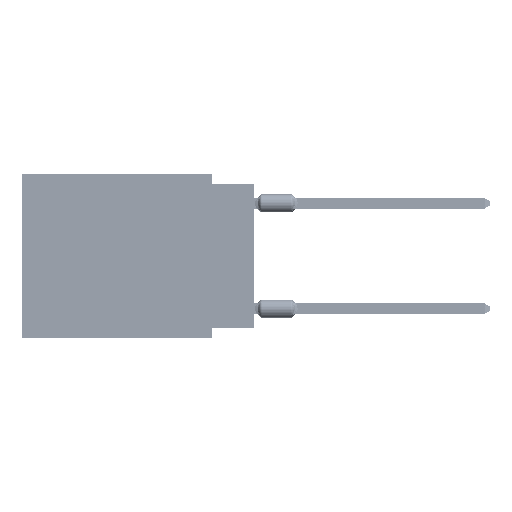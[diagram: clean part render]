
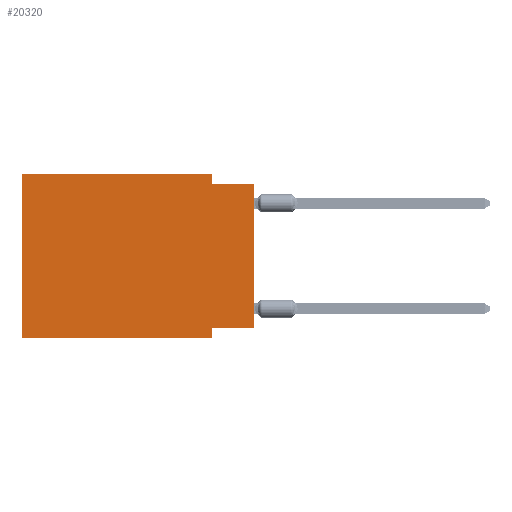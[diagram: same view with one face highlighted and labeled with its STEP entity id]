
A CAD part, left-side view. The second image highlights one B-rep face of the part: STEP entity #20320.
In plain terms, the highlighted planar face has unit normal (-1, 0, 0).
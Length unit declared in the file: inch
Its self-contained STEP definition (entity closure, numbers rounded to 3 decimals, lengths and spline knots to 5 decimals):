
#220 = DIRECTION ( 'NONE',  ( 0., -1., 0. ) ) ;
#3624 = EDGE_CURVE ( 'NONE', #69415, #12185, #21627, .T. ) ;
#5870 = EDGE_CURVE ( 'NONE', #60290, #19445, #73942, .T. ) ;
#5998 = LINE ( 'NONE', #48182, #35065 ) ;
#10390 = VECTOR ( 'NONE', #67314, 39.37008 ) ;
#12185 = VERTEX_POINT ( 'NONE', #50914 ) ;
#12834 = EDGE_CURVE ( 'NONE', #14353, #69415, #37160, .T. ) ;
#13113 = VECTOR ( 'NONE', #46015, 39.37008 ) ;
#14353 = VERTEX_POINT ( 'NONE', #72200 ) ;
#15005 = CARTESIAN_POINT ( 'NONE',  ( 0., 0.55, 0. ) ) ;
#15422 = CARTESIAN_POINT ( 'NONE',  ( 0., 0., -0.025 ) ) ;
#16132 = VECTOR ( 'NONE', #220, 39.37008 ) ;
#16364 = CARTESIAN_POINT ( 'NONE',  ( 0., 0., 0. ) ) ;
#17928 = ORIENTED_EDGE ( 'NONE', *, *, #3624, .F. ) ;
#17980 = DIRECTION ( 'NONE',  ( 0., -1., 0. ) ) ;
#18324 = CARTESIAN_POINT ( 'NONE',  ( 0., 0.1, -0.025 ) ) ;
#18380 = CARTESIAN_POINT ( 'NONE',  ( 0., 0.55, -0.39 ) ) ;
#18414 = LINE ( 'NONE', #43646, #60698 ) ;
#19445 = VERTEX_POINT ( 'NONE', #15005 ) ;
#20320 = ADVANCED_FACE ( 'NONE', ( #28320 ), #79960, .F. ) ;
#21627 = LINE ( 'NONE', #15422, #13113 ) ;
#25124 = CARTESIAN_POINT ( 'NONE',  ( 0., 0.1, -0.365 ) ) ;
#25837 = VERTEX_POINT ( 'NONE', #25124 ) ;
#26886 = ORIENTED_EDGE ( 'NONE', *, *, #46074, .F. ) ;
#28320 = FACE_OUTER_BOUND ( 'NONE', #49642, .T. ) ;
#30932 = VECTOR ( 'NONE', #67724, 39.37008 ) ;
#31060 = DIRECTION ( 'NONE',  ( 0., 1., 0. ) ) ;
#33191 = EDGE_CURVE ( 'NONE', #34754, #12185, #79596, .T. ) ;
#33242 = CARTESIAN_POINT ( 'NONE',  ( 0., 0., -0.365 ) ) ;
#34754 = VERTEX_POINT ( 'NONE', #33242 ) ;
#34957 = DIRECTION ( 'NONE',  ( 1., 0., 0. ) ) ;
#34961 = ORIENTED_EDGE ( 'NONE', *, *, #33191, .T. ) ;
#35065 = VECTOR ( 'NONE', #17980, 39.37008 ) ;
#35127 = CARTESIAN_POINT ( 'NONE',  ( 0., 0.55, 0. ) ) ;
#37160 = LINE ( 'NONE', #73938, #10390 ) ;
#38554 = EDGE_CURVE ( 'NONE', #19445, #14353, #5998, .T. ) ;
#38617 = LINE ( 'NONE', #18380, #16132 ) ;
#39394 = ORIENTED_EDGE ( 'NONE', *, *, #5870, .F. ) ;
#40020 = CARTESIAN_POINT ( 'NONE',  ( 0., 0.55, -0.39 ) ) ;
#40668 = CARTESIAN_POINT ( 'NONE',  ( 0., 0.1, -0.39 ) ) ;
#40911 = ORIENTED_EDGE ( 'NONE', *, *, #12834, .F. ) ;
#42010 = VECTOR ( 'NONE', #31060, 39.37008 ) ;
#43646 = CARTESIAN_POINT ( 'NONE',  ( 0., 0.1, -0.39 ) ) ;
#46015 = DIRECTION ( 'NONE',  ( 0., -1., 0. ) ) ;
#46074 = EDGE_CURVE ( 'NONE', #25837, #51732, #18414, .T. ) ;
#47357 = CARTESIAN_POINT ( 'NONE',  ( 0., 0.55, 0. ) ) ;
#48182 = CARTESIAN_POINT ( 'NONE',  ( 0., 0.55, 0. ) ) ;
#49642 = EDGE_LOOP ( 'NONE', ( #34961, #17928, #40911, #70899, #39394, #62776, #26886, #67715 ) ) ;
#50914 = CARTESIAN_POINT ( 'NONE',  ( 0., 0., -0.025 ) ) ;
#51732 = VERTEX_POINT ( 'NONE', #40668 ) ;
#56298 = CARTESIAN_POINT ( 'NONE',  ( 0., 0., -0.365 ) ) ;
#57003 = EDGE_CURVE ( 'NONE', #34754, #25837, #75297, .T. ) ;
#60152 = DIRECTION ( 'NONE',  ( 0., 0., -1. ) ) ;
#60290 = VERTEX_POINT ( 'NONE', #40020 ) ;
#60698 = VECTOR ( 'NONE', #62632, 39.37008 ) ;
#62632 = DIRECTION ( 'NONE',  ( 0., 0., -1. ) ) ;
#62776 = ORIENTED_EDGE ( 'NONE', *, *, #72056, .T. ) ;
#67314 = DIRECTION ( 'NONE',  ( 0., 0., -1. ) ) ;
#67715 = ORIENTED_EDGE ( 'NONE', *, *, #57003, .F. ) ;
#67724 = DIRECTION ( 'NONE',  ( 0., 0., 1. ) ) ;
#69415 = VERTEX_POINT ( 'NONE', #18324 ) ;
#70899 = ORIENTED_EDGE ( 'NONE', *, *, #38554, .F. ) ;
#72056 = EDGE_CURVE ( 'NONE', #60290, #51732, #38617, .T. ) ;
#72200 = CARTESIAN_POINT ( 'NONE',  ( 0., 0.1, 0. ) ) ;
#73938 = CARTESIAN_POINT ( 'NONE',  ( 0., 0.1, 0. ) ) ;
#73942 = LINE ( 'NONE', #35127, #30932 ) ;
#75297 = LINE ( 'NONE', #56298, #42010 ) ;
#75356 = VECTOR ( 'NONE', #78379, 39.37008 ) ;
#77895 = AXIS2_PLACEMENT_3D ( 'NONE', #47357, #34957, #60152 ) ;
#78379 = DIRECTION ( 'NONE',  ( 0., 0., 1. ) ) ;
#79596 = LINE ( 'NONE', #16364, #75356 ) ;
#79960 = PLANE ( 'NONE',  #77895 ) ;
